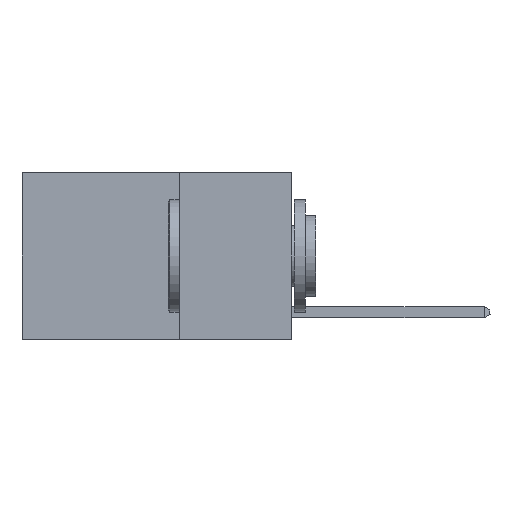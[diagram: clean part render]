
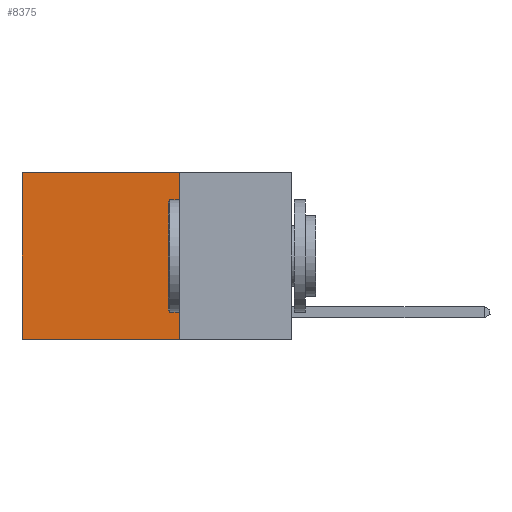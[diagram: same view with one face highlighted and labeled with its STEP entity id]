
A CAD part, left-side view. The second image highlights one B-rep face of the part: STEP entity #8375.
In plain terms, the highlighted planar face has unit normal (-1, 0, 0).
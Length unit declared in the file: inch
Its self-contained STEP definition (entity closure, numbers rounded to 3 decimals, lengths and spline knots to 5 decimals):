
#511 = PLANE ( 'NONE',  #14703 ) ;
#696 = DIRECTION ( 'NONE',  ( 0., 1., 0. ) ) ;
#1092 = EDGE_CURVE ( 'NONE', #6495, #5674, #2812, .T. ) ;
#1365 = ORIENTED_EDGE ( 'NONE', *, *, #1092, .F. ) ;
#2009 = LINE ( 'NONE', #8678, #12342 ) ;
#2055 = DIRECTION ( 'NONE',  ( 0., 0., -1. ) ) ;
#2225 = CARTESIAN_POINT ( 'NONE',  ( 0.2625, 0.25, -0.37 ) ) ;
#2812 = LINE ( 'NONE', #14766, #9945 ) ;
#3027 = CARTESIAN_POINT ( 'NONE',  ( 0.2625, 0.6, -0.37 ) ) ;
#3691 = ORIENTED_EDGE ( 'NONE', *, *, #17429, .F. ) ;
#3746 = VERTEX_POINT ( 'NONE', #11751 ) ;
#5674 = VERTEX_POINT ( 'NONE', #15880 ) ;
#5886 = VECTOR ( 'NONE', #2055, 39.37008 ) ;
#6173 = LINE ( 'NONE', #2225, #17273 ) ;
#6487 = EDGE_CURVE ( 'NONE', #3746, #6985, #13412, .T. ) ;
#6495 = VERTEX_POINT ( 'NONE', #13236 ) ;
#6704 = EDGE_CURVE ( 'NONE', #6495, #3746, #2009, .T. ) ;
#6808 = ORIENTED_EDGE ( 'NONE', *, *, #6704, .T. ) ;
#6985 = VERTEX_POINT ( 'NONE', #3027 ) ;
#8225 = EDGE_LOOP ( 'NONE', ( #10215, #3691, #1365, #6808 ) ) ;
#8375 = ADVANCED_FACE ( 'NONE', ( #8766 ), #511, .F. ) ;
#8678 = CARTESIAN_POINT ( 'NONE',  ( 0.2625, 0.25, 0. ) ) ;
#8766 = FACE_OUTER_BOUND ( 'NONE', #8225, .T. ) ;
#9945 = VECTOR ( 'NONE', #14937, 39.37008 ) ;
#10215 = ORIENTED_EDGE ( 'NONE', *, *, #6487, .T. ) ;
#11295 = DIRECTION ( 'NONE',  ( 0., 1., 0. ) ) ;
#11751 = CARTESIAN_POINT ( 'NONE',  ( 0.2625, 0.6, 0. ) ) ;
#12342 = VECTOR ( 'NONE', #696, 39.37008 ) ;
#13236 = CARTESIAN_POINT ( 'NONE',  ( 0.2625, 0.25, 0. ) ) ;
#13327 = CARTESIAN_POINT ( 'NONE',  ( 0.2625, 0.6, 0. ) ) ;
#13412 = LINE ( 'NONE', #13327, #5886 ) ;
#13838 = CARTESIAN_POINT ( 'NONE',  ( 0.2625, 0.25, 0. ) ) ;
#14019 = DIRECTION ( 'NONE',  ( 0., 0., -1. ) ) ;
#14703 = AXIS2_PLACEMENT_3D ( 'NONE', #13838, #15444, #14019 ) ;
#14766 = CARTESIAN_POINT ( 'NONE',  ( 0.2625, 0.25, 0. ) ) ;
#14937 = DIRECTION ( 'NONE',  ( 0., 0., -1. ) ) ;
#15444 = DIRECTION ( 'NONE',  ( 1., 0., 0. ) ) ;
#15880 = CARTESIAN_POINT ( 'NONE',  ( 0.2625, 0.25, -0.37 ) ) ;
#17273 = VECTOR ( 'NONE', #11295, 39.37008 ) ;
#17429 = EDGE_CURVE ( 'NONE', #5674, #6985, #6173, .T. ) ;
